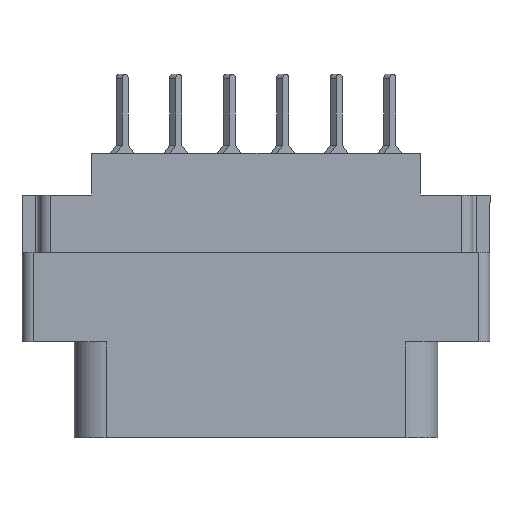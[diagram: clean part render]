
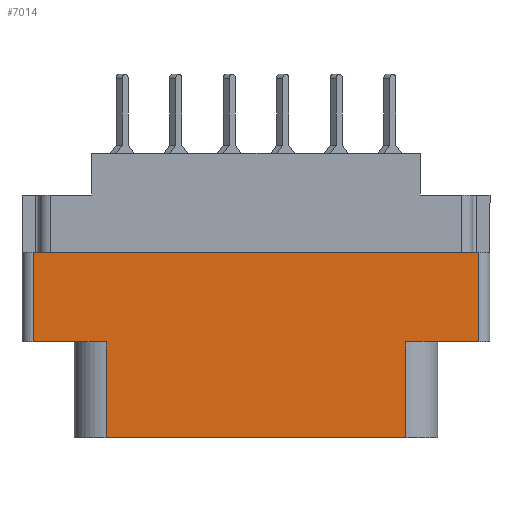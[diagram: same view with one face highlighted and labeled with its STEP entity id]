
A CAD part, front view. The second image highlights one B-rep face of the part: STEP entity #7014.
In plain terms, the highlighted planar face has unit normal (0, -1, 0).
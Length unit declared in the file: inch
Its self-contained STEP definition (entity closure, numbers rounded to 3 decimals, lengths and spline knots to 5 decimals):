
#543 = EDGE_LOOP ( 'NONE', ( #5663, #19461, #11981, #10407, #7901, #10010, #12078, #15837 ) ) ;
#794 = VERTEX_POINT ( 'NONE', #15100 ) ;
#1624 = PLANE ( 'NONE',  #10052 ) ;
#1753 = CARTESIAN_POINT ( 'NONE',  ( 0., -0.343, -0.529 ) ) ;
#1960 = LINE ( 'NONE', #3792, #9341 ) ;
#2992 = DIRECTION ( 'NONE',  ( 1., 0., 0. ) ) ;
#3152 = LINE ( 'NONE', #15518, #18488 ) ;
#3792 = CARTESIAN_POINT ( 'NONE',  ( 0., -0.343, -0.529 ) ) ;
#4532 = CARTESIAN_POINT ( 'NONE',  ( -0.624, -0.343, -0.798 ) ) ;
#4786 = DIRECTION ( 'NONE',  ( 0., 0., -1. ) ) ;
#4918 = CARTESIAN_POINT ( 'NONE',  ( 0.42, -0.343, -0.798 ) ) ;
#4989 = DIRECTION ( 'NONE',  ( 0., 0., 1. ) ) ;
#5663 = ORIENTED_EDGE ( 'NONE', *, *, #18302, .T. ) ;
#5933 = VECTOR ( 'NONE', #4786, 39.37008 ) ;
#6119 = VERTEX_POINT ( 'NONE', #19464 ) ;
#6545 = VECTOR ( 'NONE', #2992, 39.37008 ) ;
#6869 = CARTESIAN_POINT ( 'NONE',  ( 0.624, -0.343, -0.529 ) ) ;
#7014 = ADVANCED_FACE ( 'NONE', ( #11419 ), #1624, .T. ) ;
#7145 = EDGE_CURVE ( 'NONE', #6119, #9699, #18603, .T. ) ;
#7359 = LINE ( 'NONE', #14002, #5933 ) ;
#7561 = EDGE_CURVE ( 'NONE', #11495, #8809, #17401, .T. ) ;
#7901 = ORIENTED_EDGE ( 'NONE', *, *, #15513, .T. ) ;
#8809 = VERTEX_POINT ( 'NONE', #4918 ) ;
#9255 = CARTESIAN_POINT ( 'NONE',  ( -0.656, -0.343, -0.277 ) ) ;
#9341 = VECTOR ( 'NONE', #17924, 39.37008 ) ;
#9572 = LINE ( 'NONE', #19430, #14330 ) ;
#9699 = VERTEX_POINT ( 'NONE', #10153 ) ;
#9919 = CARTESIAN_POINT ( 'NONE',  ( 0.624, -0.343, -0.277 ) ) ;
#10010 = ORIENTED_EDGE ( 'NONE', *, *, #13411, .F. ) ;
#10052 = AXIS2_PLACEMENT_3D ( 'NONE', #4532, #15465, #12310 ) ;
#10153 = CARTESIAN_POINT ( 'NONE',  ( -0.624, -0.343, -0.277 ) ) ;
#10246 = VERTEX_POINT ( 'NONE', #6869 ) ;
#10407 = ORIENTED_EDGE ( 'NONE', *, *, #16744, .F. ) ;
#10942 = VECTOR ( 'NONE', #12574, 39.37008 ) ;
#11419 = FACE_OUTER_BOUND ( 'NONE', #543, .T. ) ;
#11495 = VERTEX_POINT ( 'NONE', #11702 ) ;
#11702 = CARTESIAN_POINT ( 'NONE',  ( -0.42, -0.343, -0.798 ) ) ;
#11981 = ORIENTED_EDGE ( 'NONE', *, *, #16445, .F. ) ;
#12078 = ORIENTED_EDGE ( 'NONE', *, *, #7145, .F. ) ;
#12146 = LINE ( 'NONE', #1753, #10942 ) ;
#12286 = CARTESIAN_POINT ( 'NONE',  ( -0.624, -0.343, -0.798 ) ) ;
#12310 = DIRECTION ( 'NONE',  ( 0., 0., -1. ) ) ;
#12504 = DIRECTION ( 'NONE',  ( 0., 0., -1. ) ) ;
#12574 = DIRECTION ( 'NONE',  ( 1., 0., 0. ) ) ;
#13411 = EDGE_CURVE ( 'NONE', #9699, #13669, #15429, .T. ) ;
#13593 = VECTOR ( 'NONE', #16967, 39.37008 ) ;
#13669 = VERTEX_POINT ( 'NONE', #9919 ) ;
#14002 = CARTESIAN_POINT ( 'NONE',  ( -0.42, -0.343, -0.529 ) ) ;
#14289 = CARTESIAN_POINT ( 'NONE',  ( 0.42, -0.343, -0.529 ) ) ;
#14330 = VECTOR ( 'NONE', #16571, 39.37008 ) ;
#14542 = VECTOR ( 'NONE', #4989, 39.37008 ) ;
#15100 = CARTESIAN_POINT ( 'NONE',  ( -0.42, -0.343, -0.529 ) ) ;
#15429 = LINE ( 'NONE', #9255, #6545 ) ;
#15465 = DIRECTION ( 'NONE',  ( 0., -1., 0. ) ) ;
#15513 = EDGE_CURVE ( 'NONE', #10246, #13669, #9572, .T. ) ;
#15518 = CARTESIAN_POINT ( 'NONE',  ( 0.42, -0.343, -0.529 ) ) ;
#15657 = CARTESIAN_POINT ( 'NONE',  ( -0.624, -0.343, -0.798 ) ) ;
#15837 = ORIENTED_EDGE ( 'NONE', *, *, #19227, .T. ) ;
#16445 = EDGE_CURVE ( 'NONE', #17730, #8809, #3152, .T. ) ;
#16571 = DIRECTION ( 'NONE',  ( 0., 0., 1. ) ) ;
#16744 = EDGE_CURVE ( 'NONE', #10246, #17730, #1960, .T. ) ;
#16967 = DIRECTION ( 'NONE',  ( 1., 0., 0. ) ) ;
#17401 = LINE ( 'NONE', #12286, #13593 ) ;
#17730 = VERTEX_POINT ( 'NONE', #14289 ) ;
#17924 = DIRECTION ( 'NONE',  ( -1., 0., 0. ) ) ;
#18302 = EDGE_CURVE ( 'NONE', #794, #11495, #7359, .T. ) ;
#18488 = VECTOR ( 'NONE', #12504, 39.37008 ) ;
#18603 = LINE ( 'NONE', #15657, #14542 ) ;
#19227 = EDGE_CURVE ( 'NONE', #6119, #794, #12146, .T. ) ;
#19430 = CARTESIAN_POINT ( 'NONE',  ( 0.624, -0.343, -0.798 ) ) ;
#19461 = ORIENTED_EDGE ( 'NONE', *, *, #7561, .T. ) ;
#19464 = CARTESIAN_POINT ( 'NONE',  ( -0.624, -0.343, -0.529 ) ) ;
